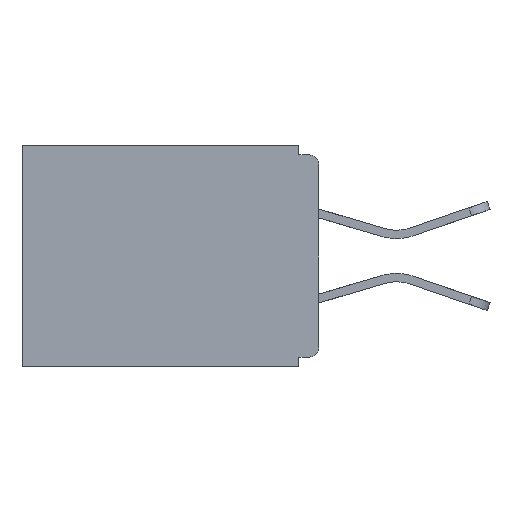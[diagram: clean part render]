
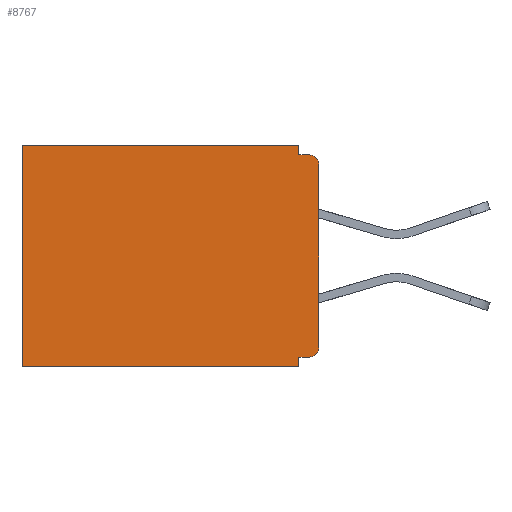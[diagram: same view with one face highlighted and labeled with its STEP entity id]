
A CAD part, left-side view. The second image highlights one B-rep face of the part: STEP entity #8767.
In plain terms, the highlighted planar face has unit normal (-1, 0, 0).
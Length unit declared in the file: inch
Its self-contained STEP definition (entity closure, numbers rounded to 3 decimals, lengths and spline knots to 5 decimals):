
#73 = VERTEX_POINT ( 'NONE', #738 ) ;
#147 = DIRECTION ( 'NONE',  ( 0., 0., -1. ) ) ;
#331 = ORIENTED_EDGE ( 'NONE', *, *, #11776, .F. ) ;
#469 = DIRECTION ( 'NONE',  ( 0., 0., -1. ) ) ;
#584 = EDGE_CURVE ( 'NONE', #8406, #7197, #6539, .T. ) ;
#604 = DIRECTION ( 'NONE',  ( 0., 0., -1. ) ) ;
#738 = CARTESIAN_POINT ( 'NONE',  ( 0.298, 0.031, -0.343 ) ) ;
#1065 = CARTESIAN_POINT ( 'NONE',  ( 0.298, 0., 0. ) ) ;
#1094 = LINE ( 'NONE', #2049, #10624 ) ;
#1101 = CARTESIAN_POINT ( 'NONE',  ( 0.298, 0.46, -0.343 ) ) ;
#1135 = CARTESIAN_POINT ( 'NONE',  ( 0.298, 0.015, -0.03 ) ) ;
#1277 = CARTESIAN_POINT ( 'NONE',  ( 0.298, 0.031, -0.328 ) ) ;
#1499 = VERTEX_POINT ( 'NONE', #8562 ) ;
#1677 = LINE ( 'NONE', #11165, #4189 ) ;
#1971 = EDGE_CURVE ( 'NONE', #1499, #2598, #4747, .T. ) ;
#2049 = CARTESIAN_POINT ( 'NONE',  ( 0.298, 0., -0.343 ) ) ;
#2213 = LINE ( 'NONE', #8995, #5944 ) ;
#2252 = VECTOR ( 'NONE', #11910, 39.37008 ) ;
#2270 = CARTESIAN_POINT ( 'NONE',  ( 0.298, 0., -0.313 ) ) ;
#2305 = ORIENTED_EDGE ( 'NONE', *, *, #1971, .T. ) ;
#2403 = CIRCLE ( 'NONE', #9314, 0.015 ) ;
#2471 = VECTOR ( 'NONE', #11290, 39.37008 ) ;
#2578 = VECTOR ( 'NONE', #6364, 39.37008 ) ;
#2598 = VERTEX_POINT ( 'NONE', #7965 ) ;
#2639 = VERTEX_POINT ( 'NONE', #10747 ) ;
#3127 = CIRCLE ( 'NONE', #4774, 0.015 ) ;
#3336 = ORIENTED_EDGE ( 'NONE', *, *, #11873, .F. ) ;
#3349 = EDGE_CURVE ( 'NONE', #73, #8231, #1094, .T. ) ;
#3435 = CARTESIAN_POINT ( 'NONE',  ( 0.298, 0.015, -0.313 ) ) ;
#3481 = LINE ( 'NONE', #4488, #2578 ) ;
#3554 = ORIENTED_EDGE ( 'NONE', *, *, #7172, .F. ) ;
#4127 = ORIENTED_EDGE ( 'NONE', *, *, #584, .F. ) ;
#4163 = CARTESIAN_POINT ( 'NONE',  ( 0.298, 0., 0. ) ) ;
#4189 = VECTOR ( 'NONE', #8864, 39.37008 ) ;
#4386 = ORIENTED_EDGE ( 'NONE', *, *, #3349, .F. ) ;
#4451 = VERTEX_POINT ( 'NONE', #1277 ) ;
#4488 = CARTESIAN_POINT ( 'NONE',  ( 0.298, 0.46, 0. ) ) ;
#4747 = LINE ( 'NONE', #1065, #7386 ) ;
#4774 = AXIS2_PLACEMENT_3D ( 'NONE', #3435, #11843, #604 ) ;
#5102 = PLANE ( 'NONE',  #5434 ) ;
#5142 = ORIENTED_EDGE ( 'NONE', *, *, #10362, .T. ) ;
#5338 = EDGE_CURVE ( 'NONE', #1499, #9214, #2213, .T. ) ;
#5434 = AXIS2_PLACEMENT_3D ( 'NONE', #4163, #11557, #10569 ) ;
#5944 = VECTOR ( 'NONE', #7083, 39.37008 ) ;
#6364 = DIRECTION ( 'NONE',  ( 0., 0., -1. ) ) ;
#6444 = ORIENTED_EDGE ( 'NONE', *, *, #5338, .F. ) ;
#6539 = LINE ( 'NONE', #10913, #2252 ) ;
#7083 = DIRECTION ( 'NONE',  ( 0., 0., -1. ) ) ;
#7089 = VERTEX_POINT ( 'NONE', #12168 ) ;
#7172 = EDGE_CURVE ( 'NONE', #2639, #4451, #7489, .T. ) ;
#7197 = VERTEX_POINT ( 'NONE', #2270 ) ;
#7386 = VECTOR ( 'NONE', #10264, 39.37008 ) ;
#7489 = LINE ( 'NONE', #7556, #2471 ) ;
#7556 = CARTESIAN_POINT ( 'NONE',  ( 0.298, 0., -0.328 ) ) ;
#7722 = DIRECTION ( 'NONE',  ( -1., 0., 0. ) ) ;
#7875 = VECTOR ( 'NONE', #147, 39.37008 ) ;
#7891 = CARTESIAN_POINT ( 'NONE',  ( 0.298, 0., -0.03 ) ) ;
#7965 = CARTESIAN_POINT ( 'NONE',  ( 0.298, 0.46, 0. ) ) ;
#8231 = VERTEX_POINT ( 'NONE', #1101 ) ;
#8406 = VERTEX_POINT ( 'NONE', #7891 ) ;
#8562 = CARTESIAN_POINT ( 'NONE',  ( 0.298, 0.031, 0. ) ) ;
#8680 = EDGE_LOOP ( 'NONE', ( #9240, #3336, #6444, #2305, #5142, #4386, #331, #3554, #9539, #4127 ) ) ;
#8767 = ADVANCED_FACE ( 'NONE', ( #12132 ), #5102, .F. ) ;
#8864 = DIRECTION ( 'NONE',  ( 0., -1., 0. ) ) ;
#8995 = CARTESIAN_POINT ( 'NONE',  ( 0.298, 0.031, -0.343 ) ) ;
#9214 = VERTEX_POINT ( 'NONE', #10298 ) ;
#9240 = ORIENTED_EDGE ( 'NONE', *, *, #11534, .T. ) ;
#9314 = AXIS2_PLACEMENT_3D ( 'NONE', #1135, #7722, #469 ) ;
#9539 = ORIENTED_EDGE ( 'NONE', *, *, #11969, .T. ) ;
#10161 = LINE ( 'NONE', #10323, #7875 ) ;
#10264 = DIRECTION ( 'NONE',  ( 0., 1., 0. ) ) ;
#10298 = CARTESIAN_POINT ( 'NONE',  ( 0.298, 0.031, -0.015 ) ) ;
#10323 = CARTESIAN_POINT ( 'NONE',  ( 0.298, 0.031, -0.343 ) ) ;
#10362 = EDGE_CURVE ( 'NONE', #2598, #8231, #3481, .T. ) ;
#10565 = DIRECTION ( 'NONE',  ( 0., 1., 0. ) ) ;
#10569 = DIRECTION ( 'NONE',  ( 0., 0., -1. ) ) ;
#10624 = VECTOR ( 'NONE', #10565, 39.37008 ) ;
#10747 = CARTESIAN_POINT ( 'NONE',  ( 0.298, 0.015, -0.328 ) ) ;
#10913 = CARTESIAN_POINT ( 'NONE',  ( 0.298, 0., 0. ) ) ;
#11165 = CARTESIAN_POINT ( 'NONE',  ( 0.298, 0., -0.015 ) ) ;
#11290 = DIRECTION ( 'NONE',  ( 0., 1., 0. ) ) ;
#11534 = EDGE_CURVE ( 'NONE', #8406, #7089, #2403, .T. ) ;
#11557 = DIRECTION ( 'NONE',  ( 1., 0., 0. ) ) ;
#11776 = EDGE_CURVE ( 'NONE', #4451, #73, #10161, .T. ) ;
#11843 = DIRECTION ( 'NONE',  ( -1., 0., 0. ) ) ;
#11873 = EDGE_CURVE ( 'NONE', #9214, #7089, #1677, .T. ) ;
#11910 = DIRECTION ( 'NONE',  ( 0., 0., -1. ) ) ;
#11969 = EDGE_CURVE ( 'NONE', #2639, #7197, #3127, .T. ) ;
#12132 = FACE_OUTER_BOUND ( 'NONE', #8680, .T. ) ;
#12168 = CARTESIAN_POINT ( 'NONE',  ( 0.298, 0.015, -0.015 ) ) ;
